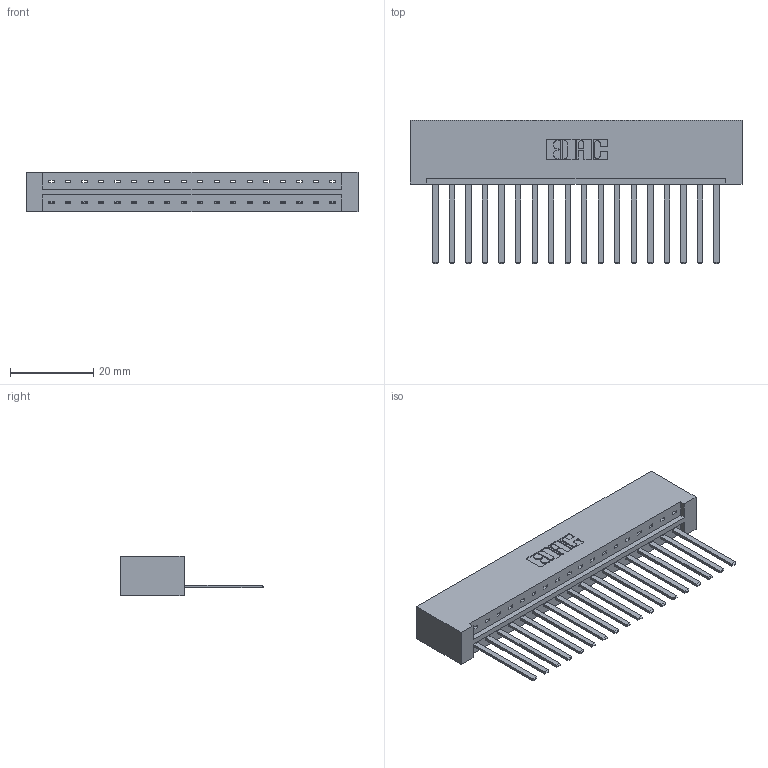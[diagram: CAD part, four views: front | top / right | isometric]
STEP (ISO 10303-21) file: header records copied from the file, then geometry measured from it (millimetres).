
FILE_DESCRIPTION (( 'STEP AP203' ), '1' );
FILE_NAME ('833-018-544-101.STEP', '2020-05-31T22:39:02', ( '' ), ( '' ), 'SwSTEP 2.0', 'SolidWorks 2020', '' );
FILE_SCHEMA (( 'CONFIG_CONTROL_DESIGN' ));
Length unit declared in the file: inch
Products named in the file (3): 345-292-001_345-293-144; 833-018-544-101; 833 Part_Lugless
Assembly tree (19 placements, depth 2):
  833-018-544-101
    833 Part_Lugless
    345-292-001_345-293-144  x18
Bounding box: 79.58 x 34.3 x 9.4 mm (x, y, z)
Volume: 8622.6 mm3; surface area: 9806.8 mm2
Topology: 19 solids, 19 shells, 1042 faces, 3131 edges, 2062 vertices
Faces by surface type: plane 750, cylinder 292
Entity records: 13647 total; most frequent: CARTESIAN_POINT 2364, ORIENTED_EDGE 2318, DIRECTION 2031, EDGE_CURVE 1159, VECTOR 1043, LINE 1043, VERTEX_POINT 770, AXIS2_PLACEMENT_3D 494
